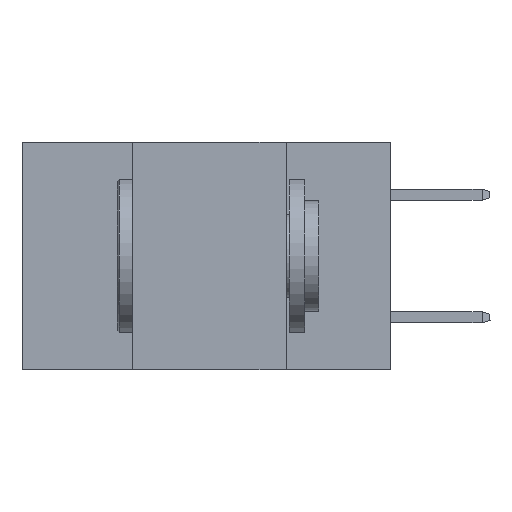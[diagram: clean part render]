
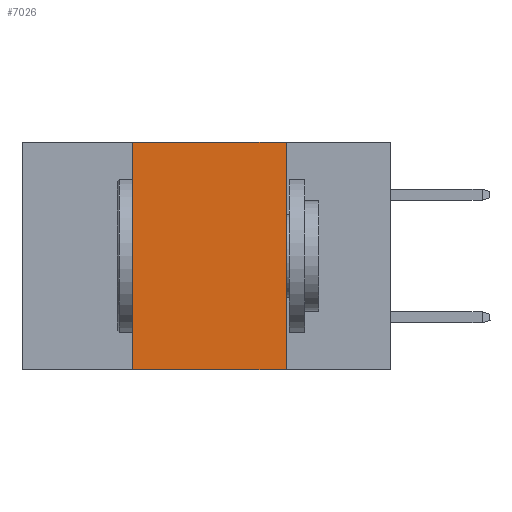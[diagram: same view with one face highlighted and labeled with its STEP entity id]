
A CAD part, left-side view. The second image highlights one B-rep face of the part: STEP entity #7026.
In plain terms, the highlighted planar face has unit normal (-1, 0, 0).
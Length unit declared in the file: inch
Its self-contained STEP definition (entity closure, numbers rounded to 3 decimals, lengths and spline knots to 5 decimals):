
#479 = CARTESIAN_POINT ( 'NONE',  ( 0., 0.17, 0. ) ) ;
#845 = PLANE ( 'NONE',  #7730 ) ;
#1344 = DIRECTION ( 'NONE',  ( 0., -1., 0. ) ) ;
#1548 = EDGE_CURVE ( 'NONE', #20805, #14897, #30075, .T. ) ;
#2337 = ORIENTED_EDGE ( 'NONE', *, *, #18737, .T. ) ;
#4859 = ORIENTED_EDGE ( 'NONE', *, *, #12288, .F. ) ;
#5663 = LINE ( 'NONE', #29606, #6469 ) ;
#6155 = LINE ( 'NONE', #479, #25770 ) ;
#6469 = VECTOR ( 'NONE', #14403, 39.37008 ) ;
#7026 = ADVANCED_FACE ( 'NONE', ( #19315 ), #845, .F. ) ;
#7730 = AXIS2_PLACEMENT_3D ( 'NONE', #20878, #30680, #18050 ) ;
#7865 = CARTESIAN_POINT ( 'NONE',  ( 0., 0.42, 0. ) ) ;
#9466 = EDGE_LOOP ( 'NONE', ( #4859, #18561, #14196, #2337 ) ) ;
#9942 = CARTESIAN_POINT ( 'NONE',  ( 0., 0.17, -0.37 ) ) ;
#12288 = EDGE_CURVE ( 'NONE', #26312, #25178, #6155, .T. ) ;
#14196 = ORIENTED_EDGE ( 'NONE', *, *, #1548, .F. ) ;
#14403 = DIRECTION ( 'NONE',  ( 0., -1., 0. ) ) ;
#14897 = VERTEX_POINT ( 'NONE', #29136 ) ;
#17052 = EDGE_CURVE ( 'NONE', #14897, #26312, #5663, .T. ) ;
#17774 = DIRECTION ( 'NONE',  ( 0., 0., -1. ) ) ;
#18050 = DIRECTION ( 'NONE',  ( 0., 0., -1. ) ) ;
#18324 = CARTESIAN_POINT ( 'NONE',  ( 0., 0.6, -0.37 ) ) ;
#18561 = ORIENTED_EDGE ( 'NONE', *, *, #17052, .F. ) ;
#18737 = EDGE_CURVE ( 'NONE', #20805, #25178, #19467, .T. ) ;
#19256 = CARTESIAN_POINT ( 'NONE',  ( 0., 0.17, 0. ) ) ;
#19315 = FACE_OUTER_BOUND ( 'NONE', #9466, .T. ) ;
#19467 = LINE ( 'NONE', #18324, #29829 ) ;
#20805 = VERTEX_POINT ( 'NONE', #24422 ) ;
#20878 = CARTESIAN_POINT ( 'NONE',  ( 0., 0.6, 0. ) ) ;
#22764 = VECTOR ( 'NONE', #22935, 39.37008 ) ;
#22935 = DIRECTION ( 'NONE',  ( 0., 0., 1. ) ) ;
#24422 = CARTESIAN_POINT ( 'NONE',  ( 0., 0.42, -0.37 ) ) ;
#25178 = VERTEX_POINT ( 'NONE', #9942 ) ;
#25770 = VECTOR ( 'NONE', #17774, 39.37008 ) ;
#26312 = VERTEX_POINT ( 'NONE', #19256 ) ;
#29136 = CARTESIAN_POINT ( 'NONE',  ( 0., 0.42, 0. ) ) ;
#29606 = CARTESIAN_POINT ( 'NONE',  ( 0., 0.6, 0. ) ) ;
#29829 = VECTOR ( 'NONE', #1344, 39.37008 ) ;
#30075 = LINE ( 'NONE', #7865, #22764 ) ;
#30680 = DIRECTION ( 'NONE',  ( 1., 0., 0. ) ) ;
